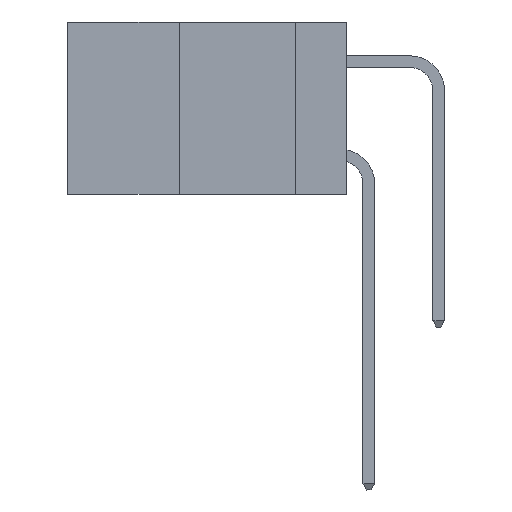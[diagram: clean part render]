
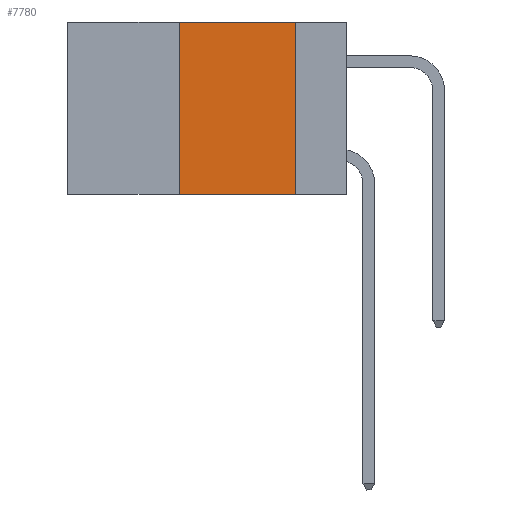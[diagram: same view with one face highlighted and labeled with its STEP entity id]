
A CAD part, left-side view. The second image highlights one B-rep face of the part: STEP entity #7780.
In plain terms, the highlighted planar face has unit normal (-1, 0, 0).
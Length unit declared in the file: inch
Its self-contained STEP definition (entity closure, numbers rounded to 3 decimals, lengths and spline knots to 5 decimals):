
#828 = ORIENTED_EDGE ( 'NONE', *, *, #11776, .F. ) ;
#975 = VECTOR ( 'NONE', #3025, 39.37008 ) ;
#1350 = VECTOR ( 'NONE', #2631, 39.37008 ) ;
#2631 = DIRECTION ( 'NONE',  ( 0., -1., 0. ) ) ;
#3025 = DIRECTION ( 'NONE',  ( 0., 0., 1. ) ) ;
#3165 = CARTESIAN_POINT ( 'NONE',  ( 0., 0.36, -0.37 ) ) ;
#3356 = VECTOR ( 'NONE', #4352, 39.37008 ) ;
#3713 = LINE ( 'NONE', #11647, #3356 ) ;
#4352 = DIRECTION ( 'NONE',  ( 0., -1., 0. ) ) ;
#4792 = EDGE_CURVE ( 'NONE', #12621, #6626, #5502, .T. ) ;
#4844 = CARTESIAN_POINT ( 'NONE',  ( 0., 0.6, 0. ) ) ;
#5224 = CARTESIAN_POINT ( 'NONE',  ( 0., 0.11, 0. ) ) ;
#5366 = EDGE_CURVE ( 'NONE', #5441, #12621, #12680, .T. ) ;
#5441 = VERTEX_POINT ( 'NONE', #8250 ) ;
#5502 = LINE ( 'NONE', #10845, #7688 ) ;
#5939 = DIRECTION ( 'NONE',  ( 0., 0., -1. ) ) ;
#5957 = CARTESIAN_POINT ( 'NONE',  ( 0., 0.6, 0. ) ) ;
#6626 = VERTEX_POINT ( 'NONE', #12694 ) ;
#6900 = EDGE_LOOP ( 'NONE', ( #9740, #10159, #828, #11606 ) ) ;
#7688 = VECTOR ( 'NONE', #9885, 39.37008 ) ;
#7780 = ADVANCED_FACE ( 'NONE', ( #13807 ), #9109, .F. ) ;
#8250 = CARTESIAN_POINT ( 'NONE',  ( 0., 0.36, 0. ) ) ;
#8494 = CARTESIAN_POINT ( 'NONE',  ( 0., 0.36, 0. ) ) ;
#9109 = PLANE ( 'NONE',  #13036 ) ;
#9740 = ORIENTED_EDGE ( 'NONE', *, *, #4792, .F. ) ;
#9885 = DIRECTION ( 'NONE',  ( 0., 0., -1. ) ) ;
#10159 = ORIENTED_EDGE ( 'NONE', *, *, #5366, .F. ) ;
#10845 = CARTESIAN_POINT ( 'NONE',  ( 0., 0.11, 0. ) ) ;
#11606 = ORIENTED_EDGE ( 'NONE', *, *, #13447, .T. ) ;
#11647 = CARTESIAN_POINT ( 'NONE',  ( 0., 0.6, -0.37 ) ) ;
#11776 = EDGE_CURVE ( 'NONE', #12767, #5441, #12084, .T. ) ;
#12084 = LINE ( 'NONE', #8494, #975 ) ;
#12092 = DIRECTION ( 'NONE',  ( 1., 0., 0. ) ) ;
#12621 = VERTEX_POINT ( 'NONE', #5224 ) ;
#12680 = LINE ( 'NONE', #5957, #1350 ) ;
#12694 = CARTESIAN_POINT ( 'NONE',  ( 0., 0.11, -0.37 ) ) ;
#12767 = VERTEX_POINT ( 'NONE', #3165 ) ;
#13036 = AXIS2_PLACEMENT_3D ( 'NONE', #4844, #12092, #5939 ) ;
#13447 = EDGE_CURVE ( 'NONE', #12767, #6626, #3713, .T. ) ;
#13807 = FACE_OUTER_BOUND ( 'NONE', #6900, .T. ) ;
